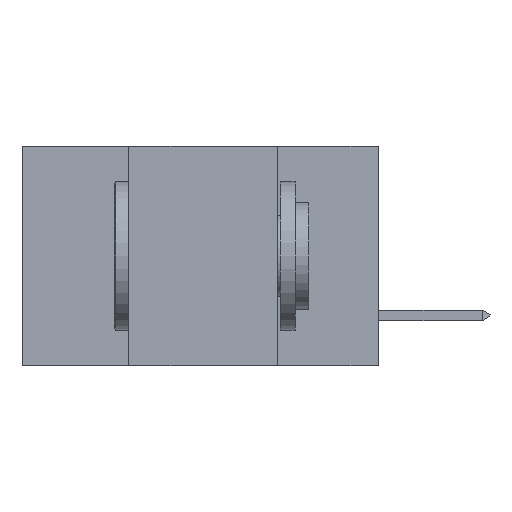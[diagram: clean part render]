
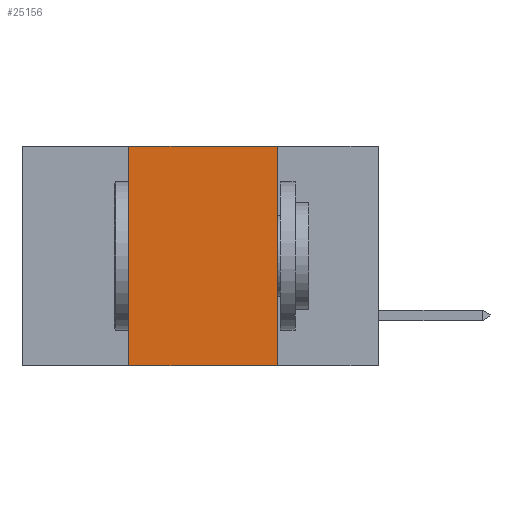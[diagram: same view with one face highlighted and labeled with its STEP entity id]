
A CAD part, left-side view. The second image highlights one B-rep face of the part: STEP entity #25156.
In plain terms, the highlighted planar face has unit normal (-1, 0, 0).
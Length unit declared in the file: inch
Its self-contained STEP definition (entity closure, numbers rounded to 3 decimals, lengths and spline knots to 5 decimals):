
#496 = LINE ( 'NONE', #25023, #10406 ) ;
#509 = DIRECTION ( 'NONE',  ( 1., 0., 0. ) ) ;
#1162 = VERTEX_POINT ( 'NONE', #3255 ) ;
#2036 = ORIENTED_EDGE ( 'NONE', *, *, #17945, .F. ) ;
#3005 = CARTESIAN_POINT ( 'NONE',  ( 0., 0.6, 0. ) ) ;
#3255 = CARTESIAN_POINT ( 'NONE',  ( 0., 0.17, -0.37 ) ) ;
#3924 = VECTOR ( 'NONE', #9569, 39.37008 ) ;
#4500 = CARTESIAN_POINT ( 'NONE',  ( 0., 0.42, 0. ) ) ;
#5089 = EDGE_LOOP ( 'NONE', ( #6349, #26218, #2036, #23181 ) ) ;
#5960 = VERTEX_POINT ( 'NONE', #4500 ) ;
#6187 = VERTEX_POINT ( 'NONE', #9716 ) ;
#6349 = ORIENTED_EDGE ( 'NONE', *, *, #11980, .F. ) ;
#8361 = VECTOR ( 'NONE', #22735, 39.37008 ) ;
#8789 = CARTESIAN_POINT ( 'NONE',  ( 0., 0.6, -0.37 ) ) ;
#9569 = DIRECTION ( 'NONE',  ( 0., -1., 0. ) ) ;
#9716 = CARTESIAN_POINT ( 'NONE',  ( 0., 0.17, 0. ) ) ;
#10268 = LINE ( 'NONE', #24784, #8361 ) ;
#10406 = VECTOR ( 'NONE', #19004, 39.37008 ) ;
#10595 = VECTOR ( 'NONE', #11367, 39.37008 ) ;
#11367 = DIRECTION ( 'NONE',  ( 0., -1., 0. ) ) ;
#11980 = EDGE_CURVE ( 'NONE', #6187, #1162, #496, .T. ) ;
#14437 = CARTESIAN_POINT ( 'NONE',  ( 0., 0.42, -0.37 ) ) ;
#15151 = DIRECTION ( 'NONE',  ( 0., 0., -1. ) ) ;
#15357 = EDGE_CURVE ( 'NONE', #16146, #1162, #21140, .T. ) ;
#16146 = VERTEX_POINT ( 'NONE', #14437 ) ;
#17945 = EDGE_CURVE ( 'NONE', #16146, #5960, #10268, .T. ) ;
#19004 = DIRECTION ( 'NONE',  ( 0., 0., -1. ) ) ;
#19017 = EDGE_CURVE ( 'NONE', #5960, #6187, #21811, .T. ) ;
#19283 = PLANE ( 'NONE',  #21087 ) ;
#21087 = AXIS2_PLACEMENT_3D ( 'NONE', #25854, #509, #15151 ) ;
#21140 = LINE ( 'NONE', #8789, #3924 ) ;
#21811 = LINE ( 'NONE', #3005, #10595 ) ;
#22735 = DIRECTION ( 'NONE',  ( 0., 0., 1. ) ) ;
#23181 = ORIENTED_EDGE ( 'NONE', *, *, #15357, .T. ) ;
#23919 = FACE_OUTER_BOUND ( 'NONE', #5089, .T. ) ;
#24784 = CARTESIAN_POINT ( 'NONE',  ( 0., 0.42, -0.37 ) ) ;
#25023 = CARTESIAN_POINT ( 'NONE',  ( 0., 0.17, -0.37 ) ) ;
#25156 = ADVANCED_FACE ( 'NONE', ( #23919 ), #19283, .F. ) ;
#25854 = CARTESIAN_POINT ( 'NONE',  ( 0., 0.6, 0. ) ) ;
#26218 = ORIENTED_EDGE ( 'NONE', *, *, #19017, .F. ) ;
